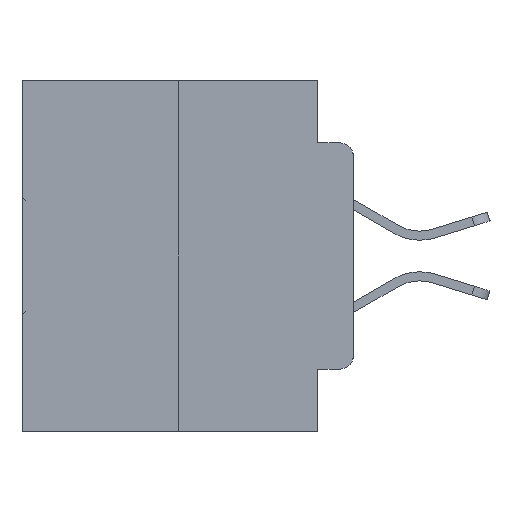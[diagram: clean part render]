
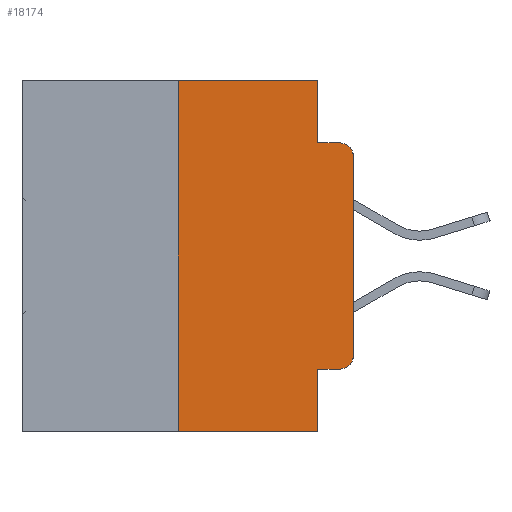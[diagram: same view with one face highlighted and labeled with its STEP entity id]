
A CAD part, left-side view. The second image highlights one B-rep face of the part: STEP entity #18174.
In plain terms, the highlighted planar face has unit normal (-1, 0, 0).
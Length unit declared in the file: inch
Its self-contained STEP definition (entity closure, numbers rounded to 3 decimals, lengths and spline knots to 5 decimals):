
#831 = DIRECTION ( 'NONE',  ( -1., 0., 0. ) ) ;
#1041 = EDGE_CURVE ( 'NONE', #24724, #5166, #28958, .T. ) ;
#2512 = CARTESIAN_POINT ( 'NONE',  ( 0., 0., 0. ) ) ;
#2711 = CARTESIAN_POINT ( 'NONE',  ( 0., 0.473, -0.5 ) ) ;
#2750 = EDGE_CURVE ( 'NONE', #21496, #5166, #9044, .T. ) ;
#2937 = CARTESIAN_POINT ( 'NONE',  ( 0., 0.051, -0.4115 ) ) ;
#3395 = CARTESIAN_POINT ( 'NONE',  ( 0., 0.051, -0.0885 ) ) ;
#4426 = EDGE_CURVE ( 'NONE', #7887, #21496, #19000, .T. ) ;
#4466 = DIRECTION ( 'NONE',  ( 0., -1., 0. ) ) ;
#4571 = DIRECTION ( 'NONE',  ( 0., 0., -1. ) ) ;
#4645 = DIRECTION ( 'NONE',  ( 0., -1., 0. ) ) ;
#4676 = CARTESIAN_POINT ( 'NONE',  ( 0., 0.02, -0.1085 ) ) ;
#4692 = VECTOR ( 'NONE', #7665, 39.37008 ) ;
#5166 = VERTEX_POINT ( 'NONE', #5170 ) ;
#5170 = CARTESIAN_POINT ( 'NONE',  ( 0., 0.02, -0.0885 ) ) ;
#5469 = LINE ( 'NONE', #2711, #4692 ) ;
#5842 = LINE ( 'NONE', #20224, #30165 ) ;
#6018 = CIRCLE ( 'NONE', #26741, 0.02 ) ;
#6279 = VECTOR ( 'NONE', #14585, 39.37008 ) ;
#6318 = EDGE_CURVE ( 'NONE', #18897, #9524, #15590, .T. ) ;
#6894 = VECTOR ( 'NONE', #11648, 39.37008 ) ;
#7064 = VECTOR ( 'NONE', #8686, 39.37008 ) ;
#7515 = DIRECTION ( 'NONE',  ( 1., 0., 0. ) ) ;
#7665 = DIRECTION ( 'NONE',  ( 0., -1., 0. ) ) ;
#7887 = VERTEX_POINT ( 'NONE', #12337 ) ;
#8686 = DIRECTION ( 'NONE',  ( 0., -1., 0. ) ) ;
#9044 = CIRCLE ( 'NONE', #10036, 0.02 ) ;
#9172 = EDGE_LOOP ( 'NONE', ( #27738, #28523, #28554, #28486, #10064, #23320, #18702, #25553, #20119, #30616 ) ) ;
#9239 = VECTOR ( 'NONE', #4466, 39.37008 ) ;
#9524 = VERTEX_POINT ( 'NONE', #23469 ) ;
#9905 = CARTESIAN_POINT ( 'NONE',  ( 0., 0.051, 0. ) ) ;
#10036 = AXIS2_PLACEMENT_3D ( 'NONE', #4676, #21348, #4571 ) ;
#10064 = ORIENTED_EDGE ( 'NONE', *, *, #6318, .F. ) ;
#11648 = DIRECTION ( 'NONE',  ( 0., 0., 1. ) ) ;
#12032 = VECTOR ( 'NONE', #14809, 39.37008 ) ;
#12337 = CARTESIAN_POINT ( 'NONE',  ( 0., 0., -0.3915 ) ) ;
#13604 = CARTESIAN_POINT ( 'NONE',  ( 0., 0.051, -0.4115 ) ) ;
#14179 = LINE ( 'NONE', #13604, #7064 ) ;
#14585 = DIRECTION ( 'NONE',  ( 0., 0., 1. ) ) ;
#14809 = DIRECTION ( 'NONE',  ( 0., 0., -1. ) ) ;
#15332 = CARTESIAN_POINT ( 'NONE',  ( 0., 0.25, -0.5 ) ) ;
#15453 = CARTESIAN_POINT ( 'NONE',  ( 0., 0.02, -0.3915 ) ) ;
#15590 = LINE ( 'NONE', #28056, #9239 ) ;
#16464 = CARTESIAN_POINT ( 'NONE',  ( 0., 0.051, -0.5 ) ) ;
#17024 = CARTESIAN_POINT ( 'NONE',  ( 0., 0.473, 0. ) ) ;
#17869 = DIRECTION ( 'NONE',  ( 0., 0., -1. ) ) ;
#18174 = ADVANCED_FACE ( 'NONE', ( #26343 ), #21697, .F. ) ;
#18620 = VERTEX_POINT ( 'NONE', #30378 ) ;
#18702 = ORIENTED_EDGE ( 'NONE', *, *, #25493, .T. ) ;
#18897 = VERTEX_POINT ( 'NONE', #22071 ) ;
#18947 = VERTEX_POINT ( 'NONE', #15332 ) ;
#19000 = LINE ( 'NONE', #2512, #6279 ) ;
#19124 = LINE ( 'NONE', #9905, #12032 ) ;
#20119 = ORIENTED_EDGE ( 'NONE', *, *, #22584, .T. ) ;
#20224 = CARTESIAN_POINT ( 'NONE',  ( 0., 0.051, 0. ) ) ;
#21019 = EDGE_CURVE ( 'NONE', #18620, #7887, #6018, .T. ) ;
#21348 = DIRECTION ( 'NONE',  ( -1., 0., 0. ) ) ;
#21496 = VERTEX_POINT ( 'NONE', #26405 ) ;
#21560 = VERTEX_POINT ( 'NONE', #2937 ) ;
#21697 = PLANE ( 'NONE',  #22208 ) ;
#22033 = VECTOR ( 'NONE', #4645, 39.37008 ) ;
#22071 = CARTESIAN_POINT ( 'NONE',  ( 0., 0.25, 0. ) ) ;
#22208 = AXIS2_PLACEMENT_3D ( 'NONE', #17024, #7515, #24055 ) ;
#22584 = EDGE_CURVE ( 'NONE', #21560, #18620, #14179, .T. ) ;
#23320 = ORIENTED_EDGE ( 'NONE', *, *, #27252, .F. ) ;
#23469 = CARTESIAN_POINT ( 'NONE',  ( 0., 0.051, 0. ) ) ;
#24055 = DIRECTION ( 'NONE',  ( 0., 0., -1. ) ) ;
#24222 = CARTESIAN_POINT ( 'NONE',  ( 0., 0.051, -0.0885 ) ) ;
#24724 = VERTEX_POINT ( 'NONE', #3395 ) ;
#24994 = LINE ( 'NONE', #25706, #6894 ) ;
#25428 = VERTEX_POINT ( 'NONE', #16464 ) ;
#25493 = EDGE_CURVE ( 'NONE', #18947, #25428, #5469, .T. ) ;
#25553 = ORIENTED_EDGE ( 'NONE', *, *, #25671, .F. ) ;
#25671 = EDGE_CURVE ( 'NONE', #21560, #25428, #5842, .T. ) ;
#25706 = CARTESIAN_POINT ( 'NONE',  ( 0., 0.25, 0. ) ) ;
#26343 = FACE_OUTER_BOUND ( 'NONE', #9172, .T. ) ;
#26405 = CARTESIAN_POINT ( 'NONE',  ( 0., 0., -0.1085 ) ) ;
#26741 = AXIS2_PLACEMENT_3D ( 'NONE', #15453, #831, #17869 ) ;
#27231 = DIRECTION ( 'NONE',  ( 0., 0., -1. ) ) ;
#27252 = EDGE_CURVE ( 'NONE', #18947, #18897, #24994, .T. ) ;
#27738 = ORIENTED_EDGE ( 'NONE', *, *, #4426, .T. ) ;
#28056 = CARTESIAN_POINT ( 'NONE',  ( 0., 0.473, 0. ) ) ;
#28486 = ORIENTED_EDGE ( 'NONE', *, *, #28803, .F. ) ;
#28523 = ORIENTED_EDGE ( 'NONE', *, *, #2750, .T. ) ;
#28554 = ORIENTED_EDGE ( 'NONE', *, *, #1041, .F. ) ;
#28803 = EDGE_CURVE ( 'NONE', #9524, #24724, #19124, .T. ) ;
#28958 = LINE ( 'NONE', #24222, #22033 ) ;
#30165 = VECTOR ( 'NONE', #27231, 39.37008 ) ;
#30378 = CARTESIAN_POINT ( 'NONE',  ( 0., 0.02, -0.4115 ) ) ;
#30616 = ORIENTED_EDGE ( 'NONE', *, *, #21019, .T. ) ;
